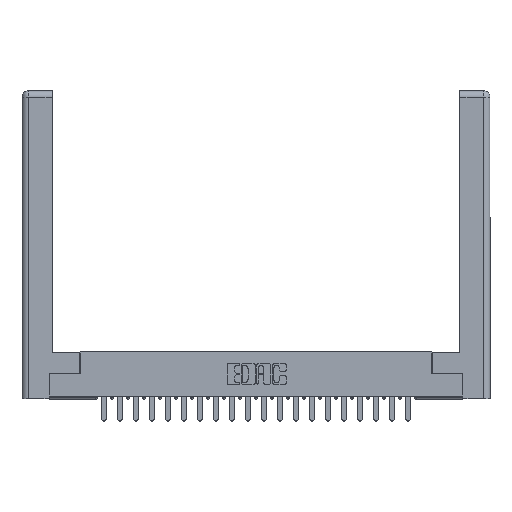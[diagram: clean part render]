
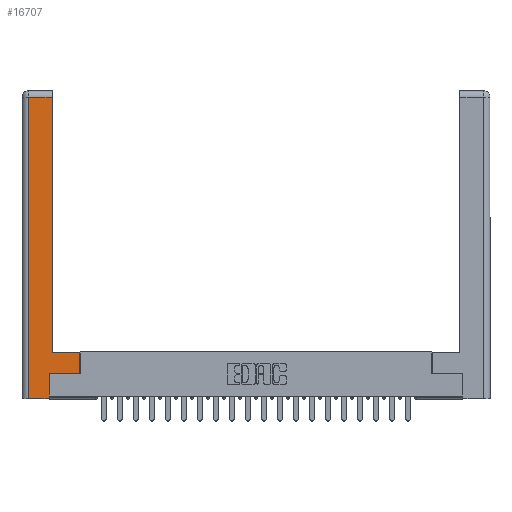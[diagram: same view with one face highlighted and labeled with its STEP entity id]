
A CAD part, top view. The second image highlights one B-rep face of the part: STEP entity #16707.
In plain terms, the highlighted planar face has unit normal (0, 0, 1).
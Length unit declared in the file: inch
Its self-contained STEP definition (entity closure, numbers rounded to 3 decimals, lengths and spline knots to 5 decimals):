
#1737 = DIRECTION ( 'NONE',  ( 1., 0., 0. ) ) ;
#2607 = LINE ( 'NONE', #17198, #26615 ) ;
#3782 = LINE ( 'NONE', #19195, #12849 ) ;
#3854 = VECTOR ( 'NONE', #16955, 39.37008 ) ;
#3886 = ORIENTED_EDGE ( 'NONE', *, *, #4218, .T. ) ;
#3953 = EDGE_CURVE ( 'NONE', #25878, #11118, #3782, .T. ) ;
#4218 = EDGE_CURVE ( 'NONE', #10725, #25499, #12503, .T. ) ;
#4387 = CARTESIAN_POINT ( 'NONE',  ( 0.295, 0.45, 0. ) ) ;
#4763 = VERTEX_POINT ( 'NONE', #5963 ) ;
#5288 = LINE ( 'NONE', #13997, #7257 ) ;
#5354 = FACE_OUTER_BOUND ( 'NONE', #9571, .T. ) ;
#5963 = CARTESIAN_POINT ( 'NONE',  ( 0.565, 0.45, 0. ) ) ;
#6013 = CARTESIAN_POINT ( 'NONE',  ( 0.265, 0., 0. ) ) ;
#6575 = LINE ( 'NONE', #12165, #15585 ) ;
#6770 = LINE ( 'NONE', #6847, #3854 ) ;
#6847 = CARTESIAN_POINT ( 'NONE',  ( 0.295, 3., 0. ) ) ;
#7257 = VECTOR ( 'NONE', #1737, 39.37008 ) ;
#7693 = CARTESIAN_POINT ( 'NONE',  ( 0.0615, 2.94, 0. ) ) ;
#7978 = ORIENTED_EDGE ( 'NONE', *, *, #26466, .T. ) ;
#8026 = VERTEX_POINT ( 'NONE', #12219 ) ;
#8413 = CARTESIAN_POINT ( 'NONE',  ( 0.0615, 2.94, 0. ) ) ;
#8865 = ORIENTED_EDGE ( 'NONE', *, *, #15095, .T. ) ;
#9258 = CARTESIAN_POINT ( 'NONE',  ( 0.295, 2.94, 0. ) ) ;
#9571 = EDGE_LOOP ( 'NONE', ( #8865, #9619, #20404, #19869, #3886, #10345, #19336, #7978 ) ) ;
#9619 = ORIENTED_EDGE ( 'NONE', *, *, #14693, .T. ) ;
#9912 = VECTOR ( 'NONE', #10545, 39.37008 ) ;
#10345 = ORIENTED_EDGE ( 'NONE', *, *, #24096, .T. ) ;
#10424 = EDGE_CURVE ( 'NONE', #8026, #4763, #2607, .T. ) ;
#10545 = DIRECTION ( 'NONE',  ( 0., 1., 0. ) ) ;
#10725 = VERTEX_POINT ( 'NONE', #6013 ) ;
#11118 = VERTEX_POINT ( 'NONE', #23649 ) ;
#11352 = LINE ( 'NONE', #22085, #18830 ) ;
#11511 = DIRECTION ( 'NONE',  ( 0., 0., -1. ) ) ;
#12165 = CARTESIAN_POINT ( 'NONE',  ( 0.265, 0., 0. ) ) ;
#12219 = CARTESIAN_POINT ( 'NONE',  ( 0.565, 0.245, 0. ) ) ;
#12503 = LINE ( 'NONE', #16835, #9912 ) ;
#12849 = VECTOR ( 'NONE', #19019, 39.37008 ) ;
#13997 = CARTESIAN_POINT ( 'NONE',  ( 0.565, 0.245, 0. ) ) ;
#14693 = EDGE_CURVE ( 'NONE', #25633, #25878, #19763, .T. ) ;
#14966 = VERTEX_POINT ( 'NONE', #4387 ) ;
#15095 = EDGE_CURVE ( 'NONE', #14966, #25633, #6770, .T. ) ;
#15585 = VECTOR ( 'NONE', #20812, 39.37008 ) ;
#15823 = CARTESIAN_POINT ( 'NONE',  ( 0., 0., 0. ) ) ;
#15874 = DIRECTION ( 'NONE',  ( -1., 0., 0. ) ) ;
#16707 = ADVANCED_FACE ( 'NONE', ( #5354 ), #24013, .F. ) ;
#16835 = CARTESIAN_POINT ( 'NONE',  ( 0.265, 0.245, 0. ) ) ;
#16955 = DIRECTION ( 'NONE',  ( 0., 1., 0. ) ) ;
#17198 = CARTESIAN_POINT ( 'NONE',  ( 0.565, 0.45, 0. ) ) ;
#18490 = VECTOR ( 'NONE', #25089, 39.37008 ) ;
#18830 = VECTOR ( 'NONE', #15874, 39.37008 ) ;
#19019 = DIRECTION ( 'NONE',  ( 0., -1., 0. ) ) ;
#19195 = CARTESIAN_POINT ( 'NONE',  ( 0.0615, 0., 0. ) ) ;
#19336 = ORIENTED_EDGE ( 'NONE', *, *, #10424, .T. ) ;
#19763 = LINE ( 'NONE', #8413, #18490 ) ;
#19869 = ORIENTED_EDGE ( 'NONE', *, *, #25279, .T. ) ;
#20404 = ORIENTED_EDGE ( 'NONE', *, *, #3953, .T. ) ;
#20679 = AXIS2_PLACEMENT_3D ( 'NONE', #15823, #11511, #22123 ) ;
#20812 = DIRECTION ( 'NONE',  ( 1., 0., 0. ) ) ;
#22085 = CARTESIAN_POINT ( 'NONE',  ( 0.295, 0.45, 0. ) ) ;
#22123 = DIRECTION ( 'NONE',  ( -1., 0., 0. ) ) ;
#23649 = CARTESIAN_POINT ( 'NONE',  ( 0.0615, 0., 0. ) ) ;
#24013 = PLANE ( 'NONE',  #20679 ) ;
#24096 = EDGE_CURVE ( 'NONE', #25499, #8026, #5288, .T. ) ;
#25089 = DIRECTION ( 'NONE',  ( -1., 0., 0. ) ) ;
#25279 = EDGE_CURVE ( 'NONE', #11118, #10725, #6575, .T. ) ;
#25307 = DIRECTION ( 'NONE',  ( 0., 1., 0. ) ) ;
#25328 = CARTESIAN_POINT ( 'NONE',  ( 0.265, 0.245, 0. ) ) ;
#25499 = VERTEX_POINT ( 'NONE', #25328 ) ;
#25633 = VERTEX_POINT ( 'NONE', #9258 ) ;
#25878 = VERTEX_POINT ( 'NONE', #7693 ) ;
#26466 = EDGE_CURVE ( 'NONE', #4763, #14966, #11352, .T. ) ;
#26615 = VECTOR ( 'NONE', #25307, 39.37008 ) ;
